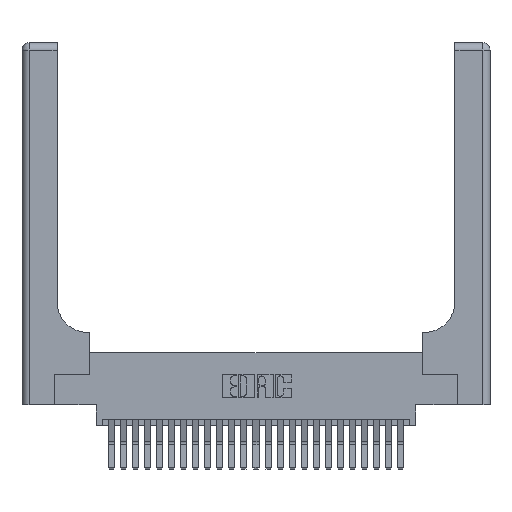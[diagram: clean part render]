
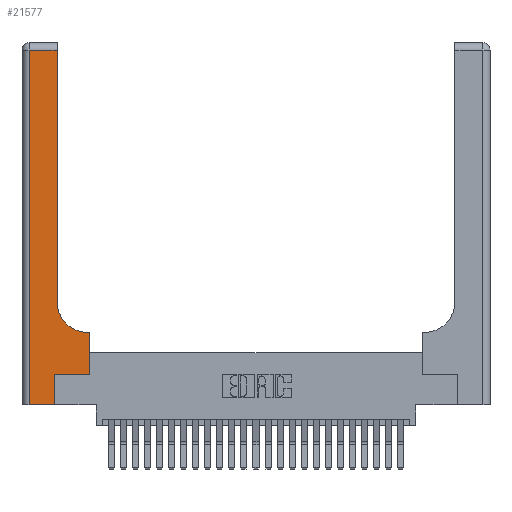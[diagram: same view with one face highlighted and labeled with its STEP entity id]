
A CAD part, top view. The second image highlights one B-rep face of the part: STEP entity #21577.
In plain terms, the highlighted planar face has unit normal (0, 0, 1).
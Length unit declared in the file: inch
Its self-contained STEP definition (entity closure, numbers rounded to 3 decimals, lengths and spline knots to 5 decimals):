
#893 = VERTEX_POINT ( 'NONE', #23664 ) ;
#1263 = AXIS2_PLACEMENT_3D ( 'NONE', #16798, #18629, #16699 ) ;
#1330 = CARTESIAN_POINT ( 'NONE',  ( 0.2915, 0.85, 0.37 ) ) ;
#1811 = ORIENTED_EDGE ( 'NONE', *, *, #20930, .T. ) ;
#1826 = EDGE_CURVE ( 'NONE', #25177, #6325, #19345, .T. ) ;
#1949 = ORIENTED_EDGE ( 'NONE', *, *, #6210, .T. ) ;
#2044 = VECTOR ( 'NONE', #9156, 39.37008 ) ;
#2194 = DIRECTION ( 'NONE',  ( -1., 0., 0. ) ) ;
#3642 = EDGE_CURVE ( 'NONE', #10466, #6718, #16969, .T. ) ;
#3885 = LINE ( 'NONE', #15424, #26645 ) ;
#4682 = DIRECTION ( 'NONE',  ( 0., -1., 0. ) ) ;
#4685 = CARTESIAN_POINT ( 'NONE',  ( 0.5585, 0.6, 0.37 ) ) ;
#6087 = CARTESIAN_POINT ( 'NONE',  ( 0.269, 0.25, 0.37 ) ) ;
#6210 = EDGE_CURVE ( 'NONE', #17947, #25053, #13903, .T. ) ;
#6325 = VERTEX_POINT ( 'NONE', #17517 ) ;
#6696 = ORIENTED_EDGE ( 'NONE', *, *, #24239, .T. ) ;
#6718 = VERTEX_POINT ( 'NONE', #15423 ) ;
#8386 = DIRECTION ( 'NONE',  ( -1., 0., 0. ) ) ;
#8554 = VECTOR ( 'NONE', #24157, 39.37008 ) ;
#9156 = DIRECTION ( 'NONE',  ( 0., 1., 0. ) ) ;
#9435 = CARTESIAN_POINT ( 'NONE',  ( 0.5585, 0.25, 0.37 ) ) ;
#9488 = VECTOR ( 'NONE', #18950, 39.37008 ) ;
#9582 = LINE ( 'NONE', #24111, #18458 ) ;
#9846 = LINE ( 'NONE', #6087, #9488 ) ;
#10131 = DIRECTION ( 'NONE',  ( 1., 0., 0. ) ) ;
#10466 = VERTEX_POINT ( 'NONE', #14224 ) ;
#12383 = EDGE_CURVE ( 'NONE', #25053, #17216, #9846, .T. ) ;
#12812 = VECTOR ( 'NONE', #10131, 39.37008 ) ;
#13764 = ORIENTED_EDGE ( 'NONE', *, *, #16535, .T. ) ;
#13903 = LINE ( 'NONE', #25546, #2044 ) ;
#14224 = CARTESIAN_POINT ( 'NONE',  ( 0.2915, 2.94, 0.37 ) ) ;
#15281 = ORIENTED_EDGE ( 'NONE', *, *, #12383, .T. ) ;
#15423 = CARTESIAN_POINT ( 'NONE',  ( 0.06, 2.94, 0.37 ) ) ;
#15424 = CARTESIAN_POINT ( 'NONE',  ( 0.06, 3., 0.37 ) ) ;
#16393 = DIRECTION ( 'NONE',  ( 1., 0., 0. ) ) ;
#16535 = EDGE_CURVE ( 'NONE', #6325, #18841, #16624, .T. ) ;
#16624 = CIRCLE ( 'NONE', #21822, 0.25 ) ;
#16699 = DIRECTION ( 'NONE',  ( -1., 0., 0. ) ) ;
#16798 = CARTESIAN_POINT ( 'NONE',  ( 0., 3., 0.37 ) ) ;
#16969 = LINE ( 'NONE', #21125, #22924 ) ;
#16988 = EDGE_LOOP ( 'NONE', ( #21870, #25029, #19924, #1811, #1949, #15281, #6696, #17098, #13764 ) ) ;
#17098 = ORIENTED_EDGE ( 'NONE', *, *, #1826, .T. ) ;
#17216 = VERTEX_POINT ( 'NONE', #25861 ) ;
#17517 = CARTESIAN_POINT ( 'NONE',  ( 0.5415, 0.6, 0.37 ) ) ;
#17678 = FACE_OUTER_BOUND ( 'NONE', #16988, .T. ) ;
#17947 = VERTEX_POINT ( 'NONE', #21712 ) ;
#18026 = DIRECTION ( 'NONE',  ( 0., 1., 0. ) ) ;
#18458 = VECTOR ( 'NONE', #18026, 39.37008 ) ;
#18629 = DIRECTION ( 'NONE',  ( 0., 0., -1. ) ) ;
#18841 = VERTEX_POINT ( 'NONE', #1330 ) ;
#18950 = DIRECTION ( 'NONE',  ( 1., 0., 0. ) ) ;
#19030 = CARTESIAN_POINT ( 'NONE',  ( 0.269, 0.25, 0.37 ) ) ;
#19345 = LINE ( 'NONE', #25202, #24650 ) ;
#19905 = EDGE_CURVE ( 'NONE', #18841, #10466, #9582, .T. ) ;
#19924 = ORIENTED_EDGE ( 'NONE', *, *, #21211, .T. ) ;
#20547 = DIRECTION ( 'NONE',  ( 0., 0., -1. ) ) ;
#20930 = EDGE_CURVE ( 'NONE', #893, #17947, #25668, .T. ) ;
#21125 = CARTESIAN_POINT ( 'NONE',  ( 0., 2.94, 0.37 ) ) ;
#21128 = PLANE ( 'NONE',  #1263 ) ;
#21211 = EDGE_CURVE ( 'NONE', #6718, #893, #3885, .T. ) ;
#21577 = ADVANCED_FACE ( 'NONE', ( #17678 ), #21128, .F. ) ;
#21712 = CARTESIAN_POINT ( 'NONE',  ( 0.269, 0., 0.37 ) ) ;
#21822 = AXIS2_PLACEMENT_3D ( 'NONE', #22831, #20547, #16393 ) ;
#21870 = ORIENTED_EDGE ( 'NONE', *, *, #19905, .T. ) ;
#22708 = CARTESIAN_POINT ( 'NONE',  ( 0., 0., 0.37 ) ) ;
#22831 = CARTESIAN_POINT ( 'NONE',  ( 0.5415, 0.85, 0.37 ) ) ;
#22924 = VECTOR ( 'NONE', #8386, 39.37008 ) ;
#23397 = LINE ( 'NONE', #9435, #8554 ) ;
#23664 = CARTESIAN_POINT ( 'NONE',  ( 0.06, 0., 0.37 ) ) ;
#24111 = CARTESIAN_POINT ( 'NONE',  ( 0.2915, 3., 0.37 ) ) ;
#24157 = DIRECTION ( 'NONE',  ( 0., 1., 0. ) ) ;
#24239 = EDGE_CURVE ( 'NONE', #17216, #25177, #23397, .T. ) ;
#24650 = VECTOR ( 'NONE', #2194, 39.37008 ) ;
#25029 = ORIENTED_EDGE ( 'NONE', *, *, #3642, .T. ) ;
#25053 = VERTEX_POINT ( 'NONE', #19030 ) ;
#25177 = VERTEX_POINT ( 'NONE', #4685 ) ;
#25202 = CARTESIAN_POINT ( 'NONE',  ( 0.2915, 0.6, 0.37 ) ) ;
#25546 = CARTESIAN_POINT ( 'NONE',  ( 0.269, 0., 0.37 ) ) ;
#25668 = LINE ( 'NONE', #22708, #12812 ) ;
#25861 = CARTESIAN_POINT ( 'NONE',  ( 0.5585, 0.25, 0.37 ) ) ;
#26645 = VECTOR ( 'NONE', #4682, 39.37008 ) ;
